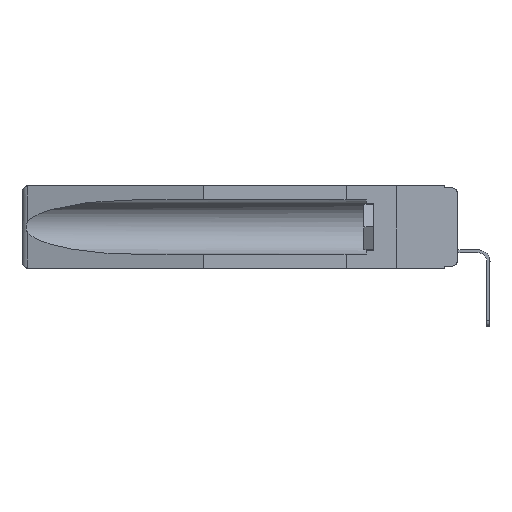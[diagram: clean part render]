
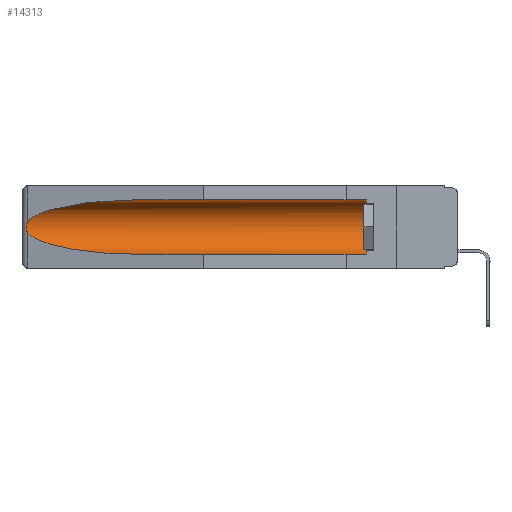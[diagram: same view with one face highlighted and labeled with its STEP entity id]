
A CAD part, left-side view. The second image highlights one B-rep face of the part: STEP entity #14313.
In plain terms, the highlighted cylindrical face has radius 2.857 mm (diameter 5.715 mm), a partial arc.
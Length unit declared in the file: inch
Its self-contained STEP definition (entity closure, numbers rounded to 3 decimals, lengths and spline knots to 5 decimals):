
#115 = EDGE_CURVE ( 'NONE', #3830, #5832, #2354, .T. ) ;
#144 =( BOUNDED_CURVE ( )  B_SPLINE_CURVE ( 3, ( #14835, #3339, #17701, #12147 ),
 .UNSPECIFIED., .F., .T. ) 
 B_SPLINE_CURVE_WITH_KNOTS ( ( 4, 4 ),
 ( 4.71239, 6.08839 ),
 .UNSPECIFIED. ) 
 CURVE ( )  GEOMETRIC_REPRESENTATION_ITEM ( )  RATIONAL_B_SPLINE_CURVE ( ( 1., 0.848, 0.848, 1. ) ) 
 REPRESENTATION_ITEM ( '' )  );
#650 = CARTESIAN_POINT ( 'NONE',  ( 0.2673, 1.53269, -0.17917 ) ) ;
#785 = CARTESIAN_POINT ( 'NONE',  ( 0.26537, 1.52718, -0.14972 ) ) ;
#793 = ORIENTED_EDGE ( 'NONE', *, *, #2689, .T. ) ;
#979 = DIRECTION ( 'NONE',  ( 0., 0., 1. ) ) ;
#2124 = CARTESIAN_POINT ( 'NONE',  ( 0.26597, 1.5296, -0.19026 ) ) ;
#2354 =( BOUNDED_CURVE ( )  B_SPLINE_CURVE ( 3, ( #2907, #14479, #15952, #7303 ),
 .UNSPECIFIED., .F., .F. ) 
 B_SPLINE_CURVE_WITH_KNOTS ( ( 4, 4 ),
 ( 0.1948, 1.5708 ),
 .UNSPECIFIED. ) 
 CURVE ( )  GEOMETRIC_REPRESENTATION_ITEM ( )  RATIONAL_B_SPLINE_CURVE ( ( 1., 0.848, 0.848, 1. ) ) 
 REPRESENTATION_ITEM ( '' )  );
#2689 = EDGE_CURVE ( 'NONE', #11701, #3830, #8291, .T. ) ;
#2907 = CARTESIAN_POINT ( 'NONE',  ( 0.26537, 1.52718, -0.19328 ) ) ;
#3339 = CARTESIAN_POINT ( 'NONE',  ( 0.21114, 1.30732, -0.059 ) ) ;
#3580 = CARTESIAN_POINT ( 'NONE',  ( 0.2673, 1.5327, -0.16383 ) ) ;
#3830 = VERTEX_POINT ( 'NONE', #9517 ) ;
#4196 = ORIENTED_EDGE ( 'NONE', *, *, #10557, .T. ) ;
#4493 = ORIENTED_EDGE ( 'NONE', *, *, #115, .T. ) ;
#5023 = CARTESIAN_POINT ( 'NONE',  ( 0.155, -0.30754, -0.284 ) ) ;
#5832 = VERTEX_POINT ( 'NONE', #7242 ) ;
#5943 = EDGE_CURVE ( 'NONE', #7336, #14287, #12843, .T. ) ;
#6050 = FACE_OUTER_BOUND ( 'NONE', #13623, .T. ) ;
#6223 = CARTESIAN_POINT ( 'NONE',  ( 0.155, -0.30754, -0.059 ) ) ;
#6432 = CARTESIAN_POINT ( 'NONE',  ( 0.155, 0.126, -0.1715 ) ) ;
#6580 = EDGE_CURVE ( 'NONE', #7840, #5832, #6965, .T. ) ;
#6965 = LINE ( 'NONE', #5023, #13941 ) ;
#7031 = EDGE_CURVE ( 'NONE', #14287, #11701, #144, .T. ) ;
#7242 = CARTESIAN_POINT ( 'NONE',  ( 0.155, 1.07973, -0.284 ) ) ;
#7303 = CARTESIAN_POINT ( 'NONE',  ( 0.155, 1.07973, -0.284 ) ) ;
#7336 = VERTEX_POINT ( 'NONE', #12699 ) ;
#7840 = VERTEX_POINT ( 'NONE', #10978 ) ;
#7910 = CARTESIAN_POINT ( 'NONE',  ( 0.2675, 1.53308, -0.16763 ) ) ;
#8209 = CARTESIAN_POINT ( 'NONE',  ( 0.155, -0.30754, -0.1715 ) ) ;
#8291 = B_SPLINE_CURVE_WITH_KNOTS ( 'NONE', 3,
 ( #785, #16547, #10922, #3580, #7910, #9343, #650, #10810, #2124, #18051 ),
 .UNSPECIFIED., .F., .F.,
 ( 4, 2, 2, 2, 4 ),
 ( 0., 0.00029, 0.00058, 0.00087, 0.00117 ),
 .UNSPECIFIED. ) ;
#8574 = VECTOR ( 'NONE', #16254, 39.37008 ) ;
#8748 = CYLINDRICAL_SURFACE ( 'NONE', #12355, 0.1125 ) ;
#9343 = CARTESIAN_POINT ( 'NONE',  ( 0.2675, 1.53308, -0.17534 ) ) ;
#9517 = CARTESIAN_POINT ( 'NONE',  ( 0.26537, 1.52718, -0.19328 ) ) ;
#9847 = ORIENTED_EDGE ( 'NONE', *, *, #6580, .F. ) ;
#10557 = EDGE_CURVE ( 'NONE', #7840, #7336, #16513, .T. ) ;
#10810 = CARTESIAN_POINT ( 'NONE',  ( 0.26655, 1.53094, -0.18657 ) ) ;
#10922 = CARTESIAN_POINT ( 'NONE',  ( 0.26654, 1.53092, -0.15636 ) ) ;
#10978 = CARTESIAN_POINT ( 'NONE',  ( 0.155, 0.126, -0.284 ) ) ;
#11236 = ORIENTED_EDGE ( 'NONE', *, *, #5943, .T. ) ;
#11701 = VERTEX_POINT ( 'NONE', #17730 ) ;
#12147 = CARTESIAN_POINT ( 'NONE',  ( 0.26537, 1.52718, -0.14972 ) ) ;
#12355 = AXIS2_PLACEMENT_3D ( 'NONE', #8209, #13939, #979 ) ;
#12633 = CARTESIAN_POINT ( 'NONE',  ( 0.155, 1.07973, -0.059 ) ) ;
#12699 = CARTESIAN_POINT ( 'NONE',  ( 0.155, 0.126, -0.059 ) ) ;
#12843 = LINE ( 'NONE', #6223, #8574 ) ;
#13623 = EDGE_LOOP ( 'NONE', ( #18199, #793, #4493, #9847, #4196, #11236 ) ) ;
#13939 = DIRECTION ( 'NONE',  ( 0., 1., 0. ) ) ;
#13941 = VECTOR ( 'NONE', #15095, 39.37008 ) ;
#14287 = VERTEX_POINT ( 'NONE', #12633 ) ;
#14313 = ADVANCED_FACE ( 'NONE', ( #6050 ), #8748, .F. ) ;
#14479 = CARTESIAN_POINT ( 'NONE',  ( 0.25451, 1.48313, -0.24835 ) ) ;
#14835 = CARTESIAN_POINT ( 'NONE',  ( 0.155, 1.07973, -0.059 ) ) ;
#15095 = DIRECTION ( 'NONE',  ( 0., 1., 0. ) ) ;
#15952 = CARTESIAN_POINT ( 'NONE',  ( 0.21114, 1.30732, -0.284 ) ) ;
#16171 = AXIS2_PLACEMENT_3D ( 'NONE', #6432, #16514, #17955 ) ;
#16254 = DIRECTION ( 'NONE',  ( 0., 1., 0. ) ) ;
#16513 = CIRCLE ( 'NONE', #16171, 0.1125 ) ;
#16514 = DIRECTION ( 'NONE',  ( 0., -1., 0. ) ) ;
#16547 = CARTESIAN_POINT ( 'NONE',  ( 0.26597, 1.52961, -0.15275 ) ) ;
#17701 = CARTESIAN_POINT ( 'NONE',  ( 0.25451, 1.48313, -0.09465 ) ) ;
#17730 = CARTESIAN_POINT ( 'NONE',  ( 0.26537, 1.52718, -0.14972 ) ) ;
#17955 = DIRECTION ( 'NONE',  ( 0., 0., 1. ) ) ;
#18051 = CARTESIAN_POINT ( 'NONE',  ( 0.26537, 1.52718, -0.19328 ) ) ;
#18199 = ORIENTED_EDGE ( 'NONE', *, *, #7031, .T. ) ;
